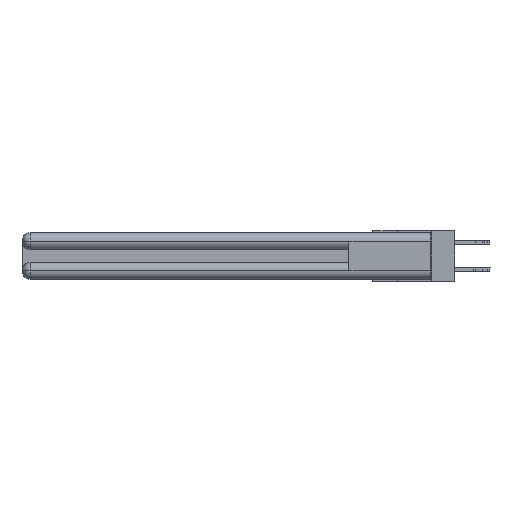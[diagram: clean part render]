
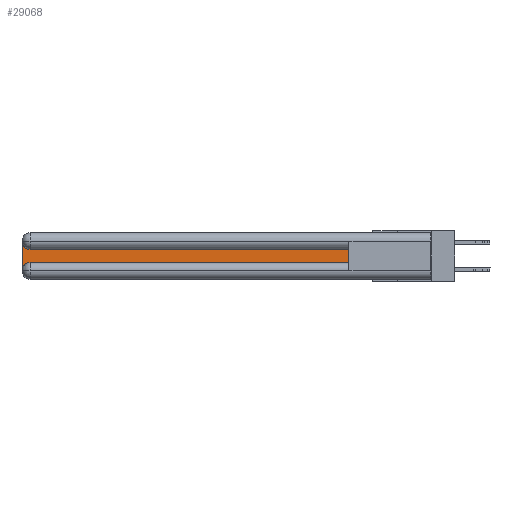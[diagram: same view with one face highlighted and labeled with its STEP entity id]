
A CAD part, left-side view. The second image highlights one B-rep face of the part: STEP entity #29068.
In plain terms, the highlighted planar face has unit normal (-1, 0, 0).
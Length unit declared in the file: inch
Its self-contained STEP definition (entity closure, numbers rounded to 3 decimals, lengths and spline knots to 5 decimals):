
#438 = EDGE_CURVE ( 'NONE', #25766, #9099, #21037, .T. ) ;
#536 = DIRECTION ( 'NONE',  ( 0., 1., 0. ) ) ;
#592 = ORIENTED_EDGE ( 'NONE', *, *, #438, .T. ) ;
#793 = ORIENTED_EDGE ( 'NONE', *, *, #19007, .T. ) ;
#1082 = LINE ( 'NONE', #9193, #23951 ) ;
#1476 = DIRECTION ( 'NONE',  ( 0., 0., 1. ) ) ;
#1707 = DIRECTION ( 'NONE',  ( 0., -1., 0. ) ) ;
#2119 = AXIS2_PLACEMENT_3D ( 'NONE', #19003, #27955, #18807 ) ;
#4016 = VECTOR ( 'NONE', #1707, 39.37008 ) ;
#4397 = ORIENTED_EDGE ( 'NONE', *, *, #21423, .T. ) ;
#5363 = LINE ( 'NONE', #6231, #22855 ) ;
#5364 = EDGE_CURVE ( 'NONE', #16519, #26996, #14858, .T. ) ;
#5575 = ORIENTED_EDGE ( 'NONE', *, *, #11282, .T. ) ;
#6172 = CARTESIAN_POINT ( 'NONE',  ( 0.075, 0.6, -0.2175 ) ) ;
#6231 = CARTESIAN_POINT ( 'NONE',  ( 0.075, 0.6, -0.2175 ) ) ;
#7364 = CARTESIAN_POINT ( 'NONE',  ( 0.075, 0.6, -0.1225 ) ) ;
#7366 = VERTEX_POINT ( 'NONE', #19577 ) ;
#9099 = VERTEX_POINT ( 'NONE', #11709 ) ;
#9193 = CARTESIAN_POINT ( 'NONE',  ( 0.075, 3., -0.2175 ) ) ;
#9761 = CARTESIAN_POINT ( 'NONE',  ( 0.075, 2.94, -0.1225 ) ) ;
#10486 = CARTESIAN_POINT ( 'NONE',  ( 0.075, 3., -0.2775 ) ) ;
#11282 = EDGE_CURVE ( 'NONE', #9099, #7366, #22594, .T. ) ;
#11709 = CARTESIAN_POINT ( 'NONE',  ( 0.075, 2.94, -0.2175 ) ) ;
#13963 = AXIS2_PLACEMENT_3D ( 'NONE', #16766, #19175, #25912 ) ;
#14056 = CARTESIAN_POINT ( 'NONE',  ( 0.075, 3., -0.0625 ) ) ;
#14858 = CIRCLE ( 'NONE', #28699, 0.06 ) ;
#15546 = CARTESIAN_POINT ( 'NONE',  ( 0.075, 0.6, -0.1225 ) ) ;
#16519 = VERTEX_POINT ( 'NONE', #9761 ) ;
#16657 = ORIENTED_EDGE ( 'NONE', *, *, #5364, .T. ) ;
#16766 = CARTESIAN_POINT ( 'NONE',  ( 0.075, 2.94, -0.2775 ) ) ;
#16941 = CARTESIAN_POINT ( 'NONE',  ( 0.075, 2.94, -0.0625 ) ) ;
#18184 = EDGE_CURVE ( 'NONE', #26996, #25766, #1082, .T. ) ;
#18278 = DIRECTION ( 'NONE',  ( 0., 0., -1. ) ) ;
#18807 = DIRECTION ( 'NONE',  ( 0., 0., -1. ) ) ;
#18904 = PLANE ( 'NONE',  #2119 ) ;
#19003 = CARTESIAN_POINT ( 'NONE',  ( 0.075, 3., -0.1225 ) ) ;
#19007 = EDGE_CURVE ( 'NONE', #7366, #22618, #5363, .T. ) ;
#19175 = DIRECTION ( 'NONE',  ( 1., 0., 0. ) ) ;
#19577 = CARTESIAN_POINT ( 'NONE',  ( 0.075, 0.6, -0.2175 ) ) ;
#20178 = EDGE_LOOP ( 'NONE', ( #4397, #16657, #27752, #592, #5575, #793 ) ) ;
#20186 = VECTOR ( 'NONE', #536, 39.37008 ) ;
#20903 = LINE ( 'NONE', #7364, #20186 ) ;
#21037 = CIRCLE ( 'NONE', #13963, 0.06 ) ;
#21423 = EDGE_CURVE ( 'NONE', #22618, #16519, #20903, .T. ) ;
#22594 = LINE ( 'NONE', #6172, #4016 ) ;
#22618 = VERTEX_POINT ( 'NONE', #15546 ) ;
#22855 = VECTOR ( 'NONE', #1476, 39.37008 ) ;
#23951 = VECTOR ( 'NONE', #18278, 39.37008 ) ;
#25766 = VERTEX_POINT ( 'NONE', #10486 ) ;
#25912 = DIRECTION ( 'NONE',  ( 0., 0., -1. ) ) ;
#26089 = DIRECTION ( 'NONE',  ( 1., 0., 0. ) ) ;
#26996 = VERTEX_POINT ( 'NONE', #14056 ) ;
#27752 = ORIENTED_EDGE ( 'NONE', *, *, #18184, .T. ) ;
#27955 = DIRECTION ( 'NONE',  ( 1., 0., 0. ) ) ;
#28434 = DIRECTION ( 'NONE',  ( 0., 0., -1. ) ) ;
#28699 = AXIS2_PLACEMENT_3D ( 'NONE', #16941, #26089, #28434 ) ;
#28802 = FACE_OUTER_BOUND ( 'NONE', #20178, .T. ) ;
#29068 = ADVANCED_FACE ( 'NONE', ( #28802 ), #18904, .F. ) ;
